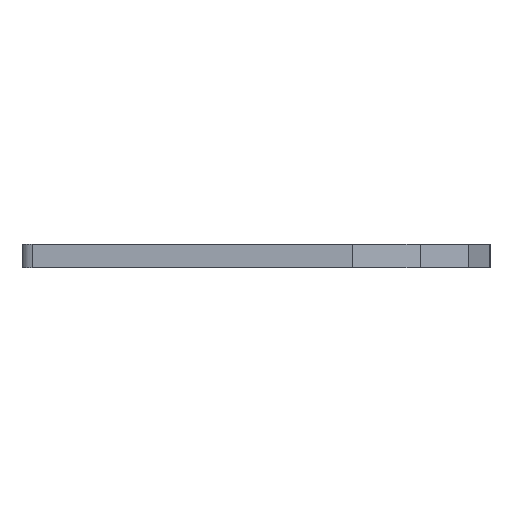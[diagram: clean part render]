
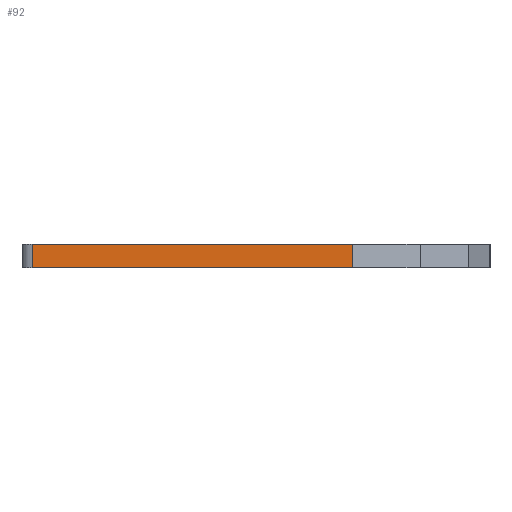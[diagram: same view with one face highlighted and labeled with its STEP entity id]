
A CAD part, left-side view. The second image highlights one B-rep face of the part: STEP entity #92.
In plain terms, the highlighted planar face has unit normal (-1, 0, 0).
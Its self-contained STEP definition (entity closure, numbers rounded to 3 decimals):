
#10 = DIRECTION ( 'NONE',  ( 0., 0., -1. ) ) ;
#92 = ADVANCED_FACE ( 'NONE', ( #1320 ), #2163, .F. ) ;
#100 = CARTESIAN_POINT ( 'NONE',  ( -90.134, -21.282, 0.203 ) ) ;
#512 = VECTOR ( 'NONE', #2227, 1000. ) ;
#555 = LINE ( 'NONE', #2267, #512 ) ;
#1002 = VERTEX_POINT ( 'NONE', #2909 ) ;
#1057 = VERTEX_POINT ( 'NONE', #2712 ) ;
#1320 = FACE_OUTER_BOUND ( 'NONE', #5062, .T. ) ;
#1479 = CARTESIAN_POINT ( 'NONE',  ( -90.134, -21.282, 0.203 ) ) ;
#1812 = VECTOR ( 'NONE', #2954, 1000. ) ;
#1837 = DIRECTION ( 'NONE',  ( 0., 0., -1. ) ) ;
#1866 = DIRECTION ( 'NONE',  ( 1., 0., 0. ) ) ;
#1927 = CARTESIAN_POINT ( 'NONE',  ( -90.134, -18.468, 0.203 ) ) ;
#1967 = ORIENTED_EDGE ( 'NONE', *, *, #4875, .T. ) ;
#1971 = ORIENTED_EDGE ( 'NONE', *, *, #4938, .F. ) ;
#1973 = ORIENTED_EDGE ( 'NONE', *, *, #3886, .F. ) ;
#1977 = ORIENTED_EDGE ( 'NONE', *, *, #4659, .T. ) ;
#2163 = PLANE ( 'NONE',  #3520 ) ;
#2227 = DIRECTION ( 'NONE',  ( 0., 0., -1. ) ) ;
#2267 = CARTESIAN_POINT ( 'NONE',  ( -90.134, -18.468, 0.203 ) ) ;
#2282 = VERTEX_POINT ( 'NONE', #1927 ) ;
#2712 = CARTESIAN_POINT ( 'NONE',  ( -90.134, -21.282, 0. ) ) ;
#2822 = VERTEX_POINT ( 'NONE', #1479 ) ;
#2909 = CARTESIAN_POINT ( 'NONE',  ( -90.134, -18.468, 0. ) ) ;
#2947 = CARTESIAN_POINT ( 'NONE',  ( -90.134, -18.468, 0.203 ) ) ;
#2954 = DIRECTION ( 'NONE',  ( 0., -1., 0. ) ) ;
#2964 = DIRECTION ( 'NONE',  ( 0., -1., 0. ) ) ;
#2970 = VECTOR ( 'NONE', #2964, 1000. ) ;
#2983 = LINE ( 'NONE', #2987, #2970 ) ;
#2987 = CARTESIAN_POINT ( 'NONE',  ( -90.134, -18.468, 0.203 ) ) ;
#3002 = CARTESIAN_POINT ( 'NONE',  ( -90.134, -18.468, 0. ) ) ;
#3520 = AXIS2_PLACEMENT_3D ( 'NONE', #2947, #1866, #1837 ) ;
#3886 = EDGE_CURVE ( 'NONE', #2282, #2822, #2983, .T. ) ;
#4621 = LINE ( 'NONE', #3002, #1812 ) ;
#4659 = EDGE_CURVE ( 'NONE', #2282, #1002, #555, .T. ) ;
#4855 = VECTOR ( 'NONE', #10, 1000. ) ;
#4875 = EDGE_CURVE ( 'NONE', #1002, #1057, #4621, .T. ) ;
#4938 = EDGE_CURVE ( 'NONE', #2822, #1057, #4964, .T. ) ;
#4964 = LINE ( 'NONE', #100, #4855 ) ;
#5062 = EDGE_LOOP ( 'NONE', ( #1967, #1971, #1973, #1977 ) ) ;
